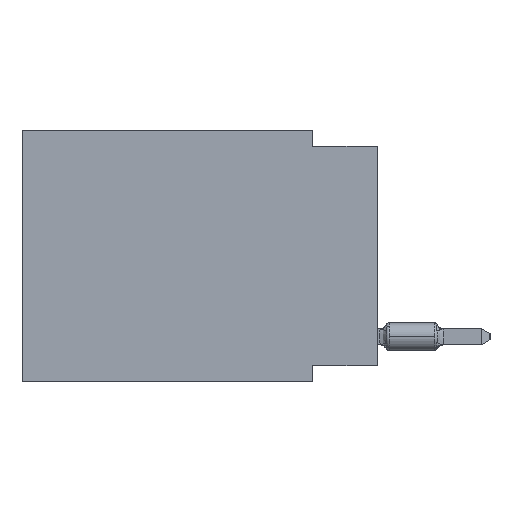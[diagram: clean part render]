
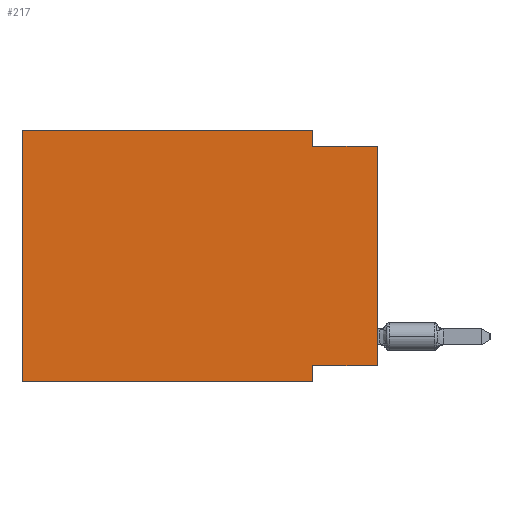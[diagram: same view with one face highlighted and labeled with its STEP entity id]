
A CAD part, left-side view. The second image highlights one B-rep face of the part: STEP entity #217.
In plain terms, the highlighted planar face has unit normal (-1, 0, 0).
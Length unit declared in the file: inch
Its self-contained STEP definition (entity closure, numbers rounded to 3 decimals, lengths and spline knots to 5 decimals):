
#217 = ADVANCED_FACE ( 'NONE', ( #42835 ), #35067, .F. ) ;
#602 = EDGE_CURVE ( 'NONE', #36729, #41578, #47450, .T. ) ;
#1388 = VERTEX_POINT ( 'NONE', #27788 ) ;
#1396 = LINE ( 'NONE', #44322, #14863 ) ;
#3320 = CARTESIAN_POINT ( 'NONE',  ( 0., 0.1, -0.39 ) ) ;
#3701 = ORIENTED_EDGE ( 'NONE', *, *, #602, .F. ) ;
#4036 = DIRECTION ( 'NONE',  ( 0., 0., -1. ) ) ;
#4241 = CARTESIAN_POINT ( 'NONE',  ( 0., 0., -0.365 ) ) ;
#4716 = CARTESIAN_POINT ( 'NONE',  ( 0., 0., -0.025 ) ) ;
#6521 = CARTESIAN_POINT ( 'NONE',  ( 0., 0.55, -0.39 ) ) ;
#7298 = EDGE_LOOP ( 'NONE', ( #28625, #34998, #21145, #3701, #37224, #20741, #48954, #26597 ) ) ;
#7904 = CARTESIAN_POINT ( 'NONE',  ( 0., 0.55, 0. ) ) ;
#8324 = DIRECTION ( 'NONE',  ( 0., 0., -1. ) ) ;
#8801 = EDGE_CURVE ( 'NONE', #21709, #43274, #37712, .T. ) ;
#10845 = VERTEX_POINT ( 'NONE', #30013 ) ;
#11783 = VECTOR ( 'NONE', #25042, 39.37008 ) ;
#12465 = LINE ( 'NONE', #16093, #25986 ) ;
#13482 = DIRECTION ( 'NONE',  ( 0., -1., 0. ) ) ;
#14863 = VECTOR ( 'NONE', #32640, 39.37008 ) ;
#16093 = CARTESIAN_POINT ( 'NONE',  ( 0., 0.1, -0.39 ) ) ;
#18010 = CARTESIAN_POINT ( 'NONE',  ( 0., 0.55, -0.39 ) ) ;
#18064 = VECTOR ( 'NONE', #13482, 39.37008 ) ;
#18878 = CARTESIAN_POINT ( 'NONE',  ( 0., 0.1, -0.365 ) ) ;
#20741 = ORIENTED_EDGE ( 'NONE', *, *, #8801, .T. ) ;
#21145 = ORIENTED_EDGE ( 'NONE', *, *, #45151, .F. ) ;
#21709 = VERTEX_POINT ( 'NONE', #6521 ) ;
#22635 = AXIS2_PLACEMENT_3D ( 'NONE', #7904, #23171, #4036 ) ;
#23171 = DIRECTION ( 'NONE',  ( 1., 0., 0. ) ) ;
#23211 = EDGE_CURVE ( 'NONE', #10845, #1388, #48176, .T. ) ;
#24663 = EDGE_CURVE ( 'NONE', #30415, #43924, #27521, .T. ) ;
#25042 = DIRECTION ( 'NONE',  ( 0., -1., 0. ) ) ;
#25986 = VECTOR ( 'NONE', #8324, 39.37008 ) ;
#26597 = ORIENTED_EDGE ( 'NONE', *, *, #24663, .F. ) ;
#26637 = CARTESIAN_POINT ( 'NONE',  ( 0., 0.55, 0. ) ) ;
#27375 = EDGE_CURVE ( 'NONE', #21709, #36729, #37141, .T. ) ;
#27521 = LINE ( 'NONE', #4241, #29752 ) ;
#27788 = CARTESIAN_POINT ( 'NONE',  ( 0., 0., -0.025 ) ) ;
#28155 = CARTESIAN_POINT ( 'NONE',  ( 0., 0.1, 0. ) ) ;
#28625 = ORIENTED_EDGE ( 'NONE', *, *, #39530, .T. ) ;
#29752 = VECTOR ( 'NONE', #31650, 39.37008 ) ;
#30013 = CARTESIAN_POINT ( 'NONE',  ( 0., 0.1, -0.025 ) ) ;
#30415 = VERTEX_POINT ( 'NONE', #43505 ) ;
#31420 = VECTOR ( 'NONE', #48354, 39.37008 ) ;
#31650 = DIRECTION ( 'NONE',  ( 0., 1., 0. ) ) ;
#32032 = LINE ( 'NONE', #28155, #31420 ) ;
#32640 = DIRECTION ( 'NONE',  ( 0., 0., 1. ) ) ;
#34998 = ORIENTED_EDGE ( 'NONE', *, *, #23211, .F. ) ;
#35067 = PLANE ( 'NONE',  #22635 ) ;
#35264 = CARTESIAN_POINT ( 'NONE',  ( 0., 0.55, 0. ) ) ;
#35894 = VECTOR ( 'NONE', #50556, 39.37008 ) ;
#36729 = VERTEX_POINT ( 'NONE', #26637 ) ;
#37141 = LINE ( 'NONE', #41538, #48157 ) ;
#37224 = ORIENTED_EDGE ( 'NONE', *, *, #27375, .F. ) ;
#37712 = LINE ( 'NONE', #18010, #11783 ) ;
#39530 = EDGE_CURVE ( 'NONE', #30415, #1388, #1396, .T. ) ;
#41538 = CARTESIAN_POINT ( 'NONE',  ( 0., 0.55, 0. ) ) ;
#41578 = VERTEX_POINT ( 'NONE', #50720 ) ;
#41795 = DIRECTION ( 'NONE',  ( 0., 0., 1. ) ) ;
#42835 = FACE_OUTER_BOUND ( 'NONE', #7298, .T. ) ;
#43274 = VERTEX_POINT ( 'NONE', #3320 ) ;
#43505 = CARTESIAN_POINT ( 'NONE',  ( 0., 0., -0.365 ) ) ;
#43924 = VERTEX_POINT ( 'NONE', #18878 ) ;
#44322 = CARTESIAN_POINT ( 'NONE',  ( 0., 0., 0. ) ) ;
#45151 = EDGE_CURVE ( 'NONE', #41578, #10845, #32032, .T. ) ;
#47450 = LINE ( 'NONE', #35264, #35894 ) ;
#48157 = VECTOR ( 'NONE', #41795, 39.37008 ) ;
#48176 = LINE ( 'NONE', #4716, #18064 ) ;
#48354 = DIRECTION ( 'NONE',  ( 0., 0., -1. ) ) ;
#48954 = ORIENTED_EDGE ( 'NONE', *, *, #51146, .F. ) ;
#50556 = DIRECTION ( 'NONE',  ( 0., -1., 0. ) ) ;
#50720 = CARTESIAN_POINT ( 'NONE',  ( 0., 0.1, 0. ) ) ;
#51146 = EDGE_CURVE ( 'NONE', #43924, #43274, #12465, .T. ) ;
